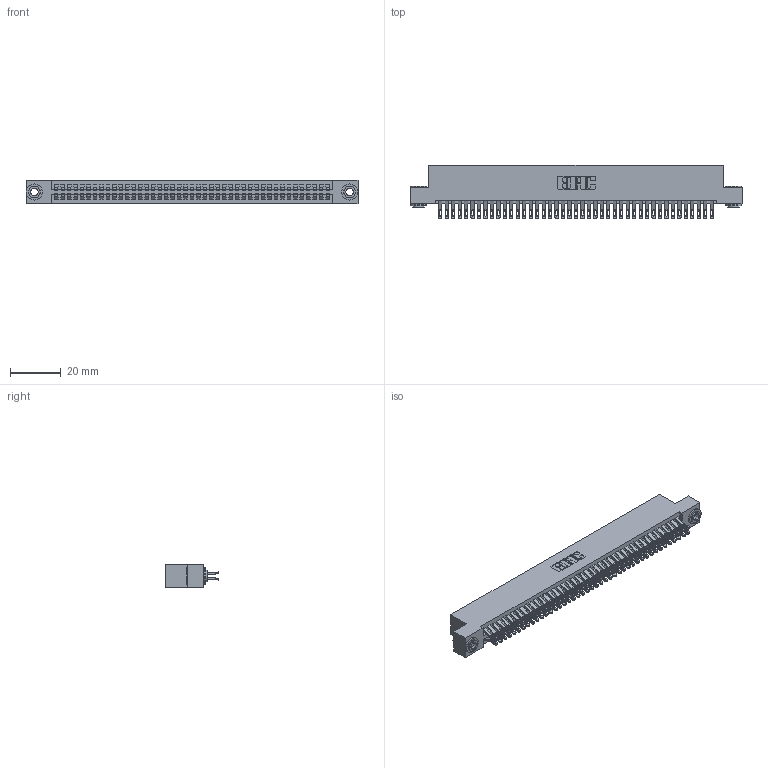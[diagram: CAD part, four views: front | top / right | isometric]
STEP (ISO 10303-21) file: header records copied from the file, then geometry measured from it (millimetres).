
FILE_DESCRIPTION (( 'STEP AP203' ), '1' );
FILE_NAME ('395-086-555-203.STEP', '2019-10-25T12:13:24', ( '' ), ( '' ), 'SwSTEP 2.0', 'SolidWorks 2016', '' );
FILE_SCHEMA (( 'CONFIG_CONTROL_DESIGN' ));
Length unit declared in the file: inch
Products named in the file (4): 345 Part_Flush Mounting Lugs - 0.156 Dia-TH; 345-292-001_555 Tail; 345-250-002_345-250-002-102; 395-086-555-203
Assembly tree (89 placements, depth 2):
  395-086-555-203
    345 Part_Flush Mounting Lugs - 0.156 Dia-TH
    345-292-001_555 Tail  x86
    345-250-002_345-250-002-102  x2
Bounding box: 130.43 x 21.13 x 9.4 mm (x, y, z)
Volume: 12948.1 mm3; surface area: 20231.4 mm2
Topology: 89 solids, 89 shells, 4980 faces, 15639 edges, 10422 vertices
Faces by surface type: plane 2756, cylinder 2216, cone 8
Entity records: 34580 total; most frequent: CARTESIAN_POINT 5805, ORIENTED_EDGE 5702, DIRECTION 5117, EDGE_CURVE 2851, LINE 2503, VECTOR 2503, VERTEX_POINT 1898, AXIS2_PLACEMENT_3D 1307
